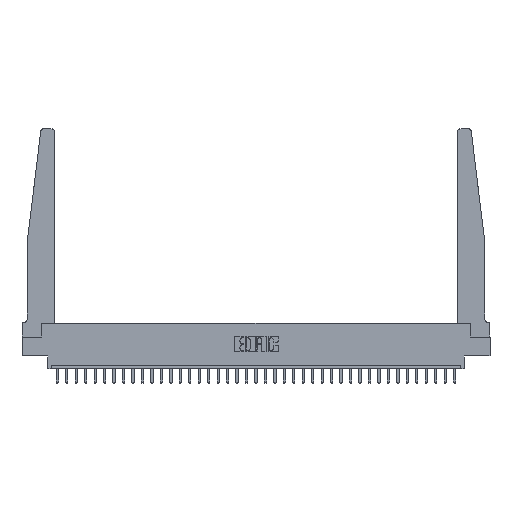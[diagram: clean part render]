
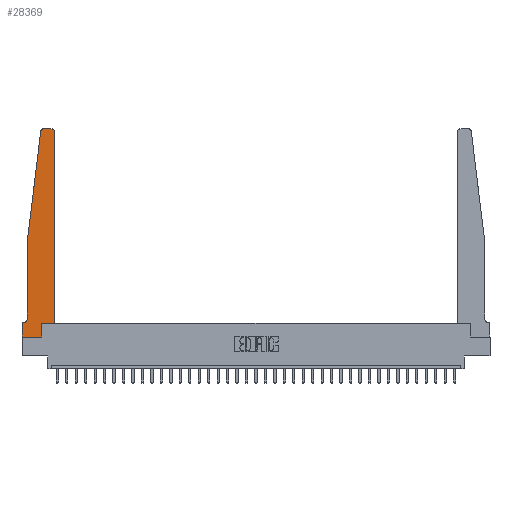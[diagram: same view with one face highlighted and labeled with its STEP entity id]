
A CAD part, top view. The second image highlights one B-rep face of the part: STEP entity #28369.
In plain terms, the highlighted planar face has unit normal (0, 0, 1).
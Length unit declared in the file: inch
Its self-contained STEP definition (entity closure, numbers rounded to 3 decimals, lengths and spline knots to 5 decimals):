
#400 = LINE ( 'NONE', #2065, #27694 ) ;
#520 = CARTESIAN_POINT ( 'NONE',  ( 0.065, 0.1875, 0.37 ) ) ;
#986 = LINE ( 'NONE', #1144, #1169 ) ;
#1044 = CIRCLE ( 'NONE', #23276, 0.05 ) ;
#1144 = CARTESIAN_POINT ( 'NONE',  ( 0.065, 1.25, 0.37 ) ) ;
#1169 = VECTOR ( 'NONE', #13146, 39.37008 ) ;
#1548 = DIRECTION ( 'NONE',  ( 0., 0., 1. ) ) ;
#2065 = CARTESIAN_POINT ( 'NONE',  ( 0., 0., 0.37 ) ) ;
#2231 = CIRCLE ( 'NONE', #29115, 0.03 ) ;
#2671 = EDGE_CURVE ( 'NONE', #5431, #5758, #7811, .T. ) ;
#2851 = DIRECTION ( 'NONE',  ( 1., 0., 0. ) ) ;
#3207 = VECTOR ( 'NONE', #14966, 39.37008 ) ;
#3224 = LINE ( 'NONE', #15718, #27384 ) ;
#3240 = EDGE_CURVE ( 'NONE', #12162, #4504, #2231, .T. ) ;
#4504 = VERTEX_POINT ( 'NONE', #28479 ) ;
#4696 = CARTESIAN_POINT ( 'NONE',  ( 0.065, 1.25, 0.37 ) ) ;
#5252 = EDGE_CURVE ( 'NONE', #9692, #5431, #1044, .T. ) ;
#5431 = VERTEX_POINT ( 'NONE', #10383 ) ;
#5758 = VERTEX_POINT ( 'NONE', #25408 ) ;
#6507 = DIRECTION ( 'NONE',  ( 0., 0., 1. ) ) ;
#6543 = EDGE_CURVE ( 'NONE', #29807, #9692, #986, .T. ) ;
#6836 = VERTEX_POINT ( 'NONE', #7286 ) ;
#7232 = PLANE ( 'NONE',  #21879 ) ;
#7286 = CARTESIAN_POINT ( 'NONE',  ( 0.425, 0.18, 0.37 ) ) ;
#7552 = VECTOR ( 'NONE', #14750, 39.37008 ) ;
#7557 = FACE_OUTER_BOUND ( 'NONE', #31265, .T. ) ;
#7811 = LINE ( 'NONE', #520, #28626 ) ;
#7970 = DIRECTION ( 'NONE',  ( -1., 0., 0. ) ) ;
#8878 = DIRECTION ( 'NONE',  ( 1., 0., 0. ) ) ;
#9018 = LINE ( 'NONE', #31193, #22281 ) ;
#9692 = VERTEX_POINT ( 'NONE', #17529 ) ;
#9956 = CIRCLE ( 'NONE', #21332, 0.03 ) ;
#9958 = EDGE_CURVE ( 'NONE', #31780, #26694, #15592, .T. ) ;
#10383 = CARTESIAN_POINT ( 'NONE',  ( 0.015, 0.1875, 0.37 ) ) ;
#11002 = DIRECTION ( 'NONE',  ( 0., 1., 0. ) ) ;
#11594 = EDGE_CURVE ( 'NONE', #6836, #29358, #3224, .T. ) ;
#11836 = ORIENTED_EDGE ( 'NONE', *, *, #22059, .T. ) ;
#11967 = VERTEX_POINT ( 'NONE', #30081 ) ;
#12162 = VERTEX_POINT ( 'NONE', #21787 ) ;
#12540 = DIRECTION ( 'NONE',  ( 1., 0., 0. ) ) ;
#13074 = EDGE_CURVE ( 'NONE', #4504, #29807, #31579, .T. ) ;
#13146 = DIRECTION ( 'NONE',  ( 0., -1., 0. ) ) ;
#13393 = EDGE_CURVE ( 'NONE', #26694, #6836, #13908, .T. ) ;
#13748 = ORIENTED_EDGE ( 'NONE', *, *, #31102, .T. ) ;
#13908 = LINE ( 'NONE', #23153, #26640 ) ;
#14529 = CARTESIAN_POINT ( 'NONE',  ( 0.425, 2.72, 0.37 ) ) ;
#14681 = VECTOR ( 'NONE', #25457, 39.37008 ) ;
#14750 = DIRECTION ( 'NONE',  ( -0.122, -0.992, 0. ) ) ;
#14966 = DIRECTION ( 'NONE',  ( 0., -1., 0. ) ) ;
#15551 = CARTESIAN_POINT ( 'NONE',  ( 0.395, 2.75, 0.37 ) ) ;
#15592 = LINE ( 'NONE', #25618, #14681 ) ;
#15718 = CARTESIAN_POINT ( 'NONE',  ( 0.425, 0.18, 0.37 ) ) ;
#16440 = CARTESIAN_POINT ( 'NONE',  ( 0.065, 1.25, 0.37 ) ) ;
#16878 = DIRECTION ( 'NONE',  ( -1., 0., 0. ) ) ;
#17117 = DIRECTION ( 'NONE',  ( 0., 0., 1. ) ) ;
#17243 = LINE ( 'NONE', #26961, #3207 ) ;
#17427 = ORIENTED_EDGE ( 'NONE', *, *, #6543, .T. ) ;
#17529 = CARTESIAN_POINT ( 'NONE',  ( 0.065, 0.2375, 0.37 ) ) ;
#18783 = CARTESIAN_POINT ( 'NONE',  ( 0.2605, 0.18, 0.37 ) ) ;
#19300 = DIRECTION ( 'NONE',  ( 0., 0., -1. ) ) ;
#20709 = ORIENTED_EDGE ( 'NONE', *, *, #5252, .T. ) ;
#21332 = AXIS2_PLACEMENT_3D ( 'NONE', #30186, #6507, #31285 ) ;
#21787 = CARTESIAN_POINT ( 'NONE',  ( 0.27653, 2.75, 0.37 ) ) ;
#21836 = ORIENTED_EDGE ( 'NONE', *, *, #2671, .T. ) ;
#21879 = AXIS2_PLACEMENT_3D ( 'NONE', #24556, #17117, #2851 ) ;
#21952 = ORIENTED_EDGE ( 'NONE', *, *, #25987, .T. ) ;
#22059 = EDGE_CURVE ( 'NONE', #28364, #12162, #9018, .T. ) ;
#22281 = VECTOR ( 'NONE', #28303, 39.37008 ) ;
#23153 = CARTESIAN_POINT ( 'NONE',  ( 0.425, 0.18, 0.37 ) ) ;
#23276 = AXIS2_PLACEMENT_3D ( 'NONE', #31594, #19300, #16878 ) ;
#23384 = ORIENTED_EDGE ( 'NONE', *, *, #11594, .T. ) ;
#24112 = EDGE_CURVE ( 'NONE', #29358, #28364, #9956, .T. ) ;
#24150 = ORIENTED_EDGE ( 'NONE', *, *, #13393, .T. ) ;
#24556 = CARTESIAN_POINT ( 'NONE',  ( 0., 0.1875, 0.37 ) ) ;
#25072 = ORIENTED_EDGE ( 'NONE', *, *, #3240, .T. ) ;
#25408 = CARTESIAN_POINT ( 'NONE',  ( 0., 0.1875, 0.37 ) ) ;
#25457 = DIRECTION ( 'NONE',  ( 0., 1., 0. ) ) ;
#25618 = CARTESIAN_POINT ( 'NONE',  ( 0.2605, 0.18, 0.37 ) ) ;
#25845 = DIRECTION ( 'NONE',  ( 1., 0., 0. ) ) ;
#25987 = EDGE_CURVE ( 'NONE', #5758, #11967, #17243, .T. ) ;
#26449 = ORIENTED_EDGE ( 'NONE', *, *, #13074, .T. ) ;
#26640 = VECTOR ( 'NONE', #8878, 39.37008 ) ;
#26694 = VERTEX_POINT ( 'NONE', #18783 ) ;
#26961 = CARTESIAN_POINT ( 'NONE',  ( 0., 0., 0.37 ) ) ;
#27384 = VECTOR ( 'NONE', #11002, 39.37008 ) ;
#27694 = VECTOR ( 'NONE', #12540, 39.37008 ) ;
#28303 = DIRECTION ( 'NONE',  ( -1., 0., 0. ) ) ;
#28364 = VERTEX_POINT ( 'NONE', #15551 ) ;
#28369 = ADVANCED_FACE ( 'NONE', ( #7557 ), #7232, .T. ) ;
#28433 = CARTESIAN_POINT ( 'NONE',  ( 0.27653, 2.72, 0.37 ) ) ;
#28479 = CARTESIAN_POINT ( 'NONE',  ( 0.24675, 2.72367, 0.37 ) ) ;
#28626 = VECTOR ( 'NONE', #7970, 39.37008 ) ;
#29115 = AXIS2_PLACEMENT_3D ( 'NONE', #28433, #1548, #25845 ) ;
#29327 = ORIENTED_EDGE ( 'NONE', *, *, #9958, .T. ) ;
#29358 = VERTEX_POINT ( 'NONE', #14529 ) ;
#29523 = ORIENTED_EDGE ( 'NONE', *, *, #24112, .T. ) ;
#29807 = VERTEX_POINT ( 'NONE', #16440 ) ;
#30081 = CARTESIAN_POINT ( 'NONE',  ( 0., 0., 0.37 ) ) ;
#30186 = CARTESIAN_POINT ( 'NONE',  ( 0.395, 2.72, 0.37 ) ) ;
#30609 = CARTESIAN_POINT ( 'NONE',  ( 0.2605, 0., 0.37 ) ) ;
#31102 = EDGE_CURVE ( 'NONE', #11967, #31780, #400, .T. ) ;
#31193 = CARTESIAN_POINT ( 'NONE',  ( 0.25, 2.75, 0.37 ) ) ;
#31265 = EDGE_LOOP ( 'NONE', ( #11836, #25072, #26449, #17427, #20709, #21836, #21952, #13748, #29327, #24150, #23384, #29523 ) ) ;
#31285 = DIRECTION ( 'NONE',  ( 1., 0., 0. ) ) ;
#31579 = LINE ( 'NONE', #4696, #7552 ) ;
#31594 = CARTESIAN_POINT ( 'NONE',  ( 0.015, 0.2375, 0.37 ) ) ;
#31780 = VERTEX_POINT ( 'NONE', #30609 ) ;
